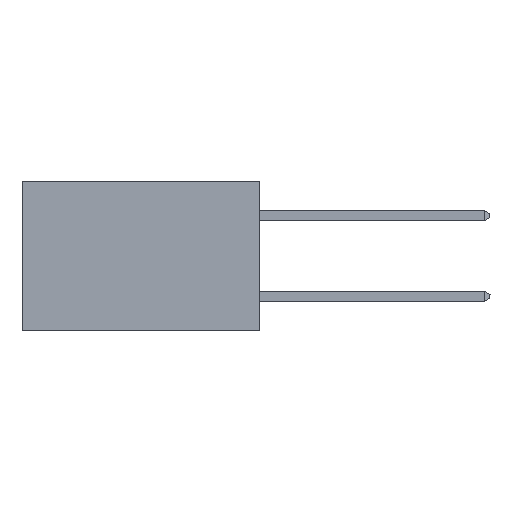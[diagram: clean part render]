
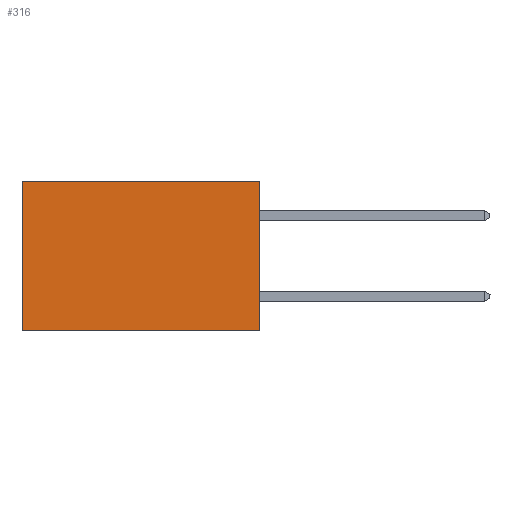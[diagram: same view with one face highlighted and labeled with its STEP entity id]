
A CAD part, left-side view. The second image highlights one B-rep face of the part: STEP entity #316.
In plain terms, the highlighted planar face has unit normal (-1, 0, 0).
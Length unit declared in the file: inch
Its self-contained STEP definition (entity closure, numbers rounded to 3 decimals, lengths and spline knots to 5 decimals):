
#26 = DIRECTION ( 'NONE',  ( 0., 0., -1. ) ) ;
#38 = DIRECTION ( 'NONE',  ( 1., 0., 0. ) ) ;
#316 = ADVANCED_FACE ( 'NONE', ( #7962 ), #5559, .F. ) ;
#1072 = VECTOR ( 'NONE', #2830, 39.37008 ) ;
#1342 = ORIENTED_EDGE ( 'NONE', *, *, #4537, .T. ) ;
#1382 = ORIENTED_EDGE ( 'NONE', *, *, #7678, .F. ) ;
#1512 = CARTESIAN_POINT ( 'NONE',  ( 0.277, 0., 0. ) ) ;
#1837 = CARTESIAN_POINT ( 'NONE',  ( 0.277, 0., 0. ) ) ;
#2071 = DIRECTION ( 'NONE',  ( 0., 0., -1. ) ) ;
#2155 = LINE ( 'NONE', #7044, #6779 ) ;
#2160 = CARTESIAN_POINT ( 'NONE',  ( 0.277, 0., -0.37 ) ) ;
#2738 = AXIS2_PLACEMENT_3D ( 'NONE', #6546, #38, #26 ) ;
#2830 = DIRECTION ( 'NONE',  ( 0., 1., 0. ) ) ;
#2886 = VERTEX_POINT ( 'NONE', #1512 ) ;
#2917 = VERTEX_POINT ( 'NONE', #7479 ) ;
#3089 = VECTOR ( 'NONE', #6528, 39.37008 ) ;
#3448 = VECTOR ( 'NONE', #6856, 39.37008 ) ;
#4252 = ORIENTED_EDGE ( 'NONE', *, *, #7743, .F. ) ;
#4415 = EDGE_LOOP ( 'NONE', ( #5596, #4252, #1382, #1342 ) ) ;
#4537 = EDGE_CURVE ( 'NONE', #2886, #2917, #7880, .T. ) ;
#4653 = EDGE_CURVE ( 'NONE', #2917, #5674, #6735, .T. ) ;
#5559 = PLANE ( 'NONE',  #2738 ) ;
#5596 = ORIENTED_EDGE ( 'NONE', *, *, #4653, .T. ) ;
#5674 = VERTEX_POINT ( 'NONE', #8019 ) ;
#5905 = CARTESIAN_POINT ( 'NONE',  ( 0.277, 0., -0.37 ) ) ;
#5994 = CARTESIAN_POINT ( 'NONE',  ( 0.277, 0.59, -0.37 ) ) ;
#6279 = LINE ( 'NONE', #2160, #1072 ) ;
#6528 = DIRECTION ( 'NONE',  ( 0., 0., -1. ) ) ;
#6546 = CARTESIAN_POINT ( 'NONE',  ( 0.277, 0., -0.37 ) ) ;
#6735 = LINE ( 'NONE', #5994, #3089 ) ;
#6779 = VECTOR ( 'NONE', #2071, 39.37008 ) ;
#6856 = DIRECTION ( 'NONE',  ( 0., 1., 0. ) ) ;
#6930 = VERTEX_POINT ( 'NONE', #5905 ) ;
#7044 = CARTESIAN_POINT ( 'NONE',  ( 0.277, 0., -0.37 ) ) ;
#7479 = CARTESIAN_POINT ( 'NONE',  ( 0.277, 0.59, 0. ) ) ;
#7678 = EDGE_CURVE ( 'NONE', #2886, #6930, #2155, .T. ) ;
#7743 = EDGE_CURVE ( 'NONE', #6930, #5674, #6279, .T. ) ;
#7880 = LINE ( 'NONE', #1837, #3448 ) ;
#7962 = FACE_OUTER_BOUND ( 'NONE', #4415, .T. ) ;
#8019 = CARTESIAN_POINT ( 'NONE',  ( 0.277, 0.59, -0.37 ) ) ;
